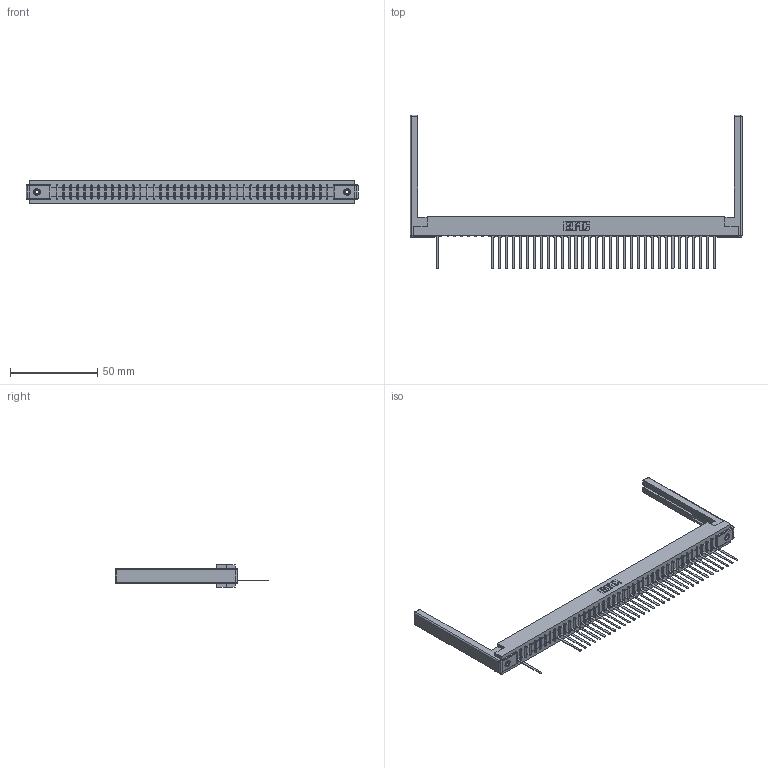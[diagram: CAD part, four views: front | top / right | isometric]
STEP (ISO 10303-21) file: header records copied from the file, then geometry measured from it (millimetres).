
FILE_DESCRIPTION (( 'STEP AP203' ), '1' );
FILE_NAME ('307-041-545-168.STEP', '2018-08-05T15:47:28', ( '' ), ( '' ), 'SwSTEP 2.0', 'SolidWorks 2016', '' );
FILE_SCHEMA (( 'CONFIG_CONTROL_DESIGN' ));
Length unit declared in the file: inch
Products named in the file (5): 307-220-068; 345-250-001_345-250-001-102; 307-041-545-168; 307 Part_.156 Dia Mounting Holes; 307-290-001_545
Assembly tree (39 placements, depth 2):
  307-041-545-168
    307 Part_.156 Dia Mounting Holes
    307-290-001_545  x34
    307-220-068  x2
    345-250-001_345-250-001-102  x2
Bounding box: 189.89 x 87.96 x 12.7 mm (x, y, z)
Volume: 24136 mm3; surface area: 25197.7 mm2
Topology: 39 solids, 39 shells, 2358 faces, 6669 edges, 4266 vertices
Faces by surface type: plane 1500, cylinder 750, sphere 92, cone 12, torus 4
Entity records: 37775 total; most frequent: CARTESIAN_POINT 6358, ORIENTED_EDGE 6340, DIRECTION 6194, EDGE_CURVE 3170, LINE 2430, VECTOR 2430, VERTEX_POINT 2046, AXIS2_PLACEMENT_3D 1882
